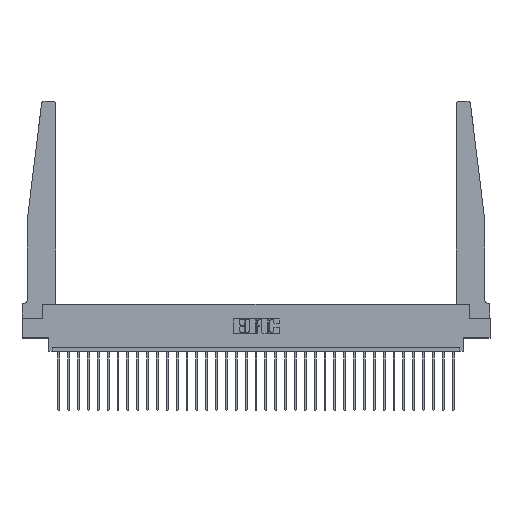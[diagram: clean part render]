
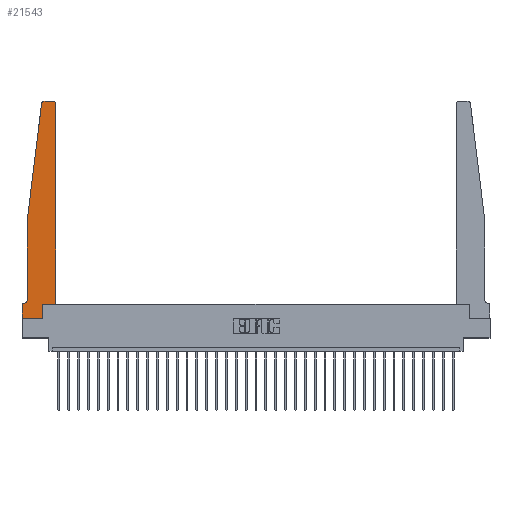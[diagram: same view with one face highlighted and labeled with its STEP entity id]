
A CAD part, top view. The second image highlights one B-rep face of the part: STEP entity #21543.
In plain terms, the highlighted planar face has unit normal (0, 0, 1).
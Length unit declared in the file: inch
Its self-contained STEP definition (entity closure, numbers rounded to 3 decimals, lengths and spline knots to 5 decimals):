
#274 = ORIENTED_EDGE ( 'NONE', *, *, #18396, .T. ) ;
#1059 = EDGE_CURVE ( 'NONE', #25063, #23305, #27008, .T. ) ;
#1594 = ORIENTED_EDGE ( 'NONE', *, *, #25036, .T. ) ;
#1752 = LINE ( 'NONE', #20684, #17403 ) ;
#1817 = CARTESIAN_POINT ( 'NONE',  ( 0.395, 2.72, 0.37 ) ) ;
#2720 = CARTESIAN_POINT ( 'NONE',  ( 0.2605, 0.18, 0.37 ) ) ;
#3243 = CARTESIAN_POINT ( 'NONE',  ( 0.395, 2.75, 0.37 ) ) ;
#3828 = CARTESIAN_POINT ( 'NONE',  ( 0.425, 0.18, 0.37 ) ) ;
#4148 = DIRECTION ( 'NONE',  ( 1., 0., 0. ) ) ;
#4593 = DIRECTION ( 'NONE',  ( 0., -1., 0. ) ) ;
#4885 = EDGE_CURVE ( 'NONE', #28101, #9340, #17162, .T. ) ;
#6027 = DIRECTION ( 'NONE',  ( 0., 1., 0. ) ) ;
#6143 = AXIS2_PLACEMENT_3D ( 'NONE', #1817, #9011, #23252 ) ;
#6345 = CARTESIAN_POINT ( 'NONE',  ( 0.425, 0.18, 0.37 ) ) ;
#6741 = VERTEX_POINT ( 'NONE', #22968 ) ;
#6877 = LINE ( 'NONE', #30506, #30482 ) ;
#7049 = EDGE_CURVE ( 'NONE', #9954, #10476, #13145, .T. ) ;
#7111 = CARTESIAN_POINT ( 'NONE',  ( 0.065, 1.25, 0.37 ) ) ;
#7404 = CARTESIAN_POINT ( 'NONE',  ( 0.27653, 2.75, 0.37 ) ) ;
#7667 = VERTEX_POINT ( 'NONE', #26346 ) ;
#8026 = ORIENTED_EDGE ( 'NONE', *, *, #4885, .T. ) ;
#8070 = CARTESIAN_POINT ( 'NONE',  ( 0.065, 0.2375, 0.37 ) ) ;
#8369 = LINE ( 'NONE', #25435, #26034 ) ;
#8468 = DIRECTION ( 'NONE',  ( 1., 0., 0. ) ) ;
#8881 = ORIENTED_EDGE ( 'NONE', *, *, #20320, .T. ) ;
#8913 = VECTOR ( 'NONE', #8468, 39.37008 ) ;
#9011 = DIRECTION ( 'NONE',  ( 0., 0., 1. ) ) ;
#9107 = EDGE_CURVE ( 'NONE', #19671, #7667, #6877, .T. ) ;
#9169 = CARTESIAN_POINT ( 'NONE',  ( 0.065, 0.1875, 0.37 ) ) ;
#9340 = VERTEX_POINT ( 'NONE', #12199 ) ;
#9413 = ORIENTED_EDGE ( 'NONE', *, *, #1059, .T. ) ;
#9469 = ORIENTED_EDGE ( 'NONE', *, *, #7049, .T. ) ;
#9763 = LINE ( 'NONE', #14621, #20217 ) ;
#9954 = VERTEX_POINT ( 'NONE', #19150 ) ;
#10476 = VERTEX_POINT ( 'NONE', #3243 ) ;
#10694 = CARTESIAN_POINT ( 'NONE',  ( 0., 0., 0.37 ) ) ;
#11121 = VECTOR ( 'NONE', #4148, 39.37008 ) ;
#11269 = DIRECTION ( 'NONE',  ( 0., 0., 1. ) ) ;
#12199 = CARTESIAN_POINT ( 'NONE',  ( 0.24675, 2.72367, 0.37 ) ) ;
#12212 = VERTEX_POINT ( 'NONE', #8070 ) ;
#12965 = CARTESIAN_POINT ( 'NONE',  ( 0., 0.1875, 0.37 ) ) ;
#13048 = DIRECTION ( 'NONE',  ( -1., 0., 0. ) ) ;
#13061 = CIRCLE ( 'NONE', #18039, 0.05 ) ;
#13103 = AXIS2_PLACEMENT_3D ( 'NONE', #12965, #22033, #21882 ) ;
#13145 = CIRCLE ( 'NONE', #6143, 0.03 ) ;
#13771 = DIRECTION ( 'NONE',  ( 1., 0., 0. ) ) ;
#14004 = EDGE_CURVE ( 'NONE', #10476, #28101, #1752, .T. ) ;
#14621 = CARTESIAN_POINT ( 'NONE',  ( 0.425, 0.18, 0.37 ) ) ;
#15074 = EDGE_LOOP ( 'NONE', ( #24539, #8026, #8881, #26369, #24764, #1594, #21692, #15327, #274, #9413, #21745, #9469 ) ) ;
#15305 = EDGE_CURVE ( 'NONE', #6741, #12212, #23530, .T. ) ;
#15327 = ORIENTED_EDGE ( 'NONE', *, *, #15533, .T. ) ;
#15533 = EDGE_CURVE ( 'NONE', #7667, #16913, #27403, .T. ) ;
#16913 = VERTEX_POINT ( 'NONE', #23267 ) ;
#17162 = CIRCLE ( 'NONE', #26676, 0.03 ) ;
#17403 = VECTOR ( 'NONE', #18328, 39.37008 ) ;
#17726 = CARTESIAN_POINT ( 'NONE',  ( 0.015, 0.2375, 0.37 ) ) ;
#18039 = AXIS2_PLACEMENT_3D ( 'NONE', #17726, #27272, #13048 ) ;
#18113 = VECTOR ( 'NONE', #28521, 39.37008 ) ;
#18328 = DIRECTION ( 'NONE',  ( -1., 0., 0. ) ) ;
#18387 = CARTESIAN_POINT ( 'NONE',  ( 0., 0.1875, 0.37 ) ) ;
#18396 = EDGE_CURVE ( 'NONE', #16913, #25063, #8369, .T. ) ;
#18829 = EDGE_CURVE ( 'NONE', #12212, #21125, #13061, .T. ) ;
#18972 = LINE ( 'NONE', #28059, #18113 ) ;
#19150 = CARTESIAN_POINT ( 'NONE',  ( 0.425, 2.72, 0.37 ) ) ;
#19671 = VERTEX_POINT ( 'NONE', #18387 ) ;
#20217 = VECTOR ( 'NONE', #26500, 39.37008 ) ;
#20320 = EDGE_CURVE ( 'NONE', #9340, #6741, #18972, .T. ) ;
#20684 = CARTESIAN_POINT ( 'NONE',  ( 0.25, 2.75, 0.37 ) ) ;
#21125 = VERTEX_POINT ( 'NONE', #24114 ) ;
#21543 = ADVANCED_FACE ( 'NONE', ( #27193 ), #22196, .T. ) ;
#21692 = ORIENTED_EDGE ( 'NONE', *, *, #9107, .T. ) ;
#21745 = ORIENTED_EDGE ( 'NONE', *, *, #24479, .T. ) ;
#21882 = DIRECTION ( 'NONE',  ( 1., 0., 0. ) ) ;
#22033 = DIRECTION ( 'NONE',  ( 0., 0., 1. ) ) ;
#22196 = PLANE ( 'NONE',  #13103 ) ;
#22247 = VECTOR ( 'NONE', #28257, 39.37008 ) ;
#22968 = CARTESIAN_POINT ( 'NONE',  ( 0.065, 1.25, 0.37 ) ) ;
#23252 = DIRECTION ( 'NONE',  ( 1., 0., 0. ) ) ;
#23267 = CARTESIAN_POINT ( 'NONE',  ( 0.2605, 0., 0.37 ) ) ;
#23305 = VERTEX_POINT ( 'NONE', #3828 ) ;
#23530 = LINE ( 'NONE', #7111, #24904 ) ;
#23551 = LINE ( 'NONE', #9169, #22247 ) ;
#24114 = CARTESIAN_POINT ( 'NONE',  ( 0.015, 0.1875, 0.37 ) ) ;
#24479 = EDGE_CURVE ( 'NONE', #23305, #9954, #9763, .T. ) ;
#24539 = ORIENTED_EDGE ( 'NONE', *, *, #14004, .T. ) ;
#24764 = ORIENTED_EDGE ( 'NONE', *, *, #18829, .T. ) ;
#24904 = VECTOR ( 'NONE', #4593, 39.37008 ) ;
#25036 = EDGE_CURVE ( 'NONE', #21125, #19671, #23551, .T. ) ;
#25063 = VERTEX_POINT ( 'NONE', #2720 ) ;
#25326 = CARTESIAN_POINT ( 'NONE',  ( 0.27653, 2.72, 0.37 ) ) ;
#25435 = CARTESIAN_POINT ( 'NONE',  ( 0.2605, 0.18, 0.37 ) ) ;
#26034 = VECTOR ( 'NONE', #6027, 39.37008 ) ;
#26346 = CARTESIAN_POINT ( 'NONE',  ( 0., 0., 0.37 ) ) ;
#26369 = ORIENTED_EDGE ( 'NONE', *, *, #15305, .T. ) ;
#26500 = DIRECTION ( 'NONE',  ( 0., 1., 0. ) ) ;
#26676 = AXIS2_PLACEMENT_3D ( 'NONE', #25326, #11269, #13771 ) ;
#27008 = LINE ( 'NONE', #6345, #11121 ) ;
#27193 = FACE_OUTER_BOUND ( 'NONE', #15074, .T. ) ;
#27272 = DIRECTION ( 'NONE',  ( 0., 0., -1. ) ) ;
#27403 = LINE ( 'NONE', #10694, #8913 ) ;
#28059 = CARTESIAN_POINT ( 'NONE',  ( 0.065, 1.25, 0.37 ) ) ;
#28101 = VERTEX_POINT ( 'NONE', #7404 ) ;
#28257 = DIRECTION ( 'NONE',  ( -1., 0., 0. ) ) ;
#28463 = DIRECTION ( 'NONE',  ( 0., -1., 0. ) ) ;
#28521 = DIRECTION ( 'NONE',  ( -0.122, -0.992, 0. ) ) ;
#30482 = VECTOR ( 'NONE', #28463, 39.37008 ) ;
#30506 = CARTESIAN_POINT ( 'NONE',  ( 0., 0., 0.37 ) ) ;
